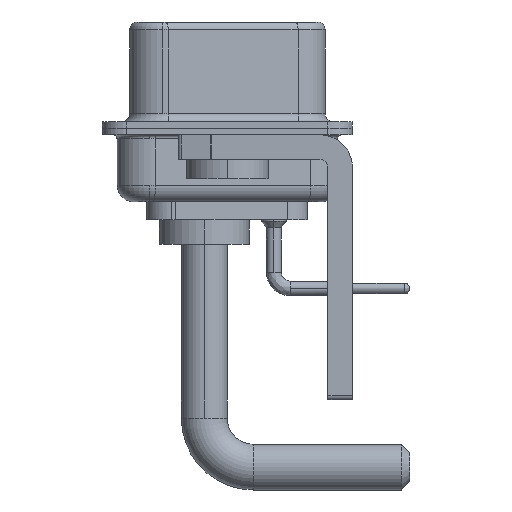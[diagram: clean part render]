
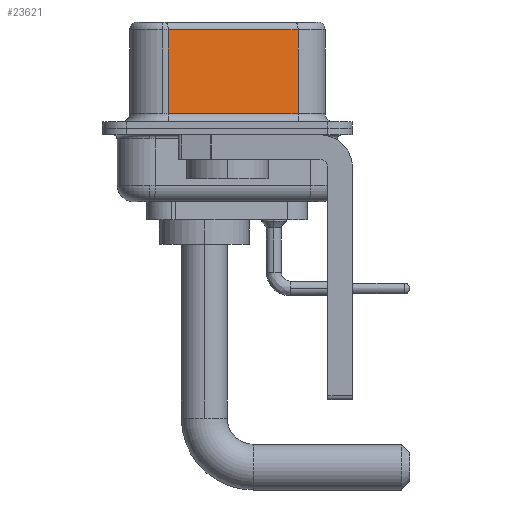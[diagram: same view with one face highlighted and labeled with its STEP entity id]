
A CAD part, left-side view. The second image highlights one B-rep face of the part: STEP entity #23621.
In plain terms, the highlighted planar face has unit normal (-0.985, -0.174, 0).
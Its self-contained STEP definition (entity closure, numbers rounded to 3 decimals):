
#509 = EDGE_CURVE ( 'NONE', #24397, #3879, #18357, .T. ) ;
#616 = CARTESIAN_POINT ( 'NONE',  ( 5.132, -4.322, 6.52 ) ) ;
#2607 = LINE ( 'NONE', #21674, #2951 ) ;
#2951 = VECTOR ( 'NONE', #10233, 1000. ) ;
#3073 = EDGE_CURVE ( 'NONE', #24397, #13013, #17763, .T. ) ;
#3879 = VERTEX_POINT ( 'NONE', #23460 ) ;
#5129 = DIRECTION ( 'NONE',  ( -0.174, 0.985, 0. ) ) ;
#5248 = CARTESIAN_POINT ( 'NONE',  ( 5.132, -4.322, 6.02 ) ) ;
#5534 = DIRECTION ( 'NONE',  ( 0., 0., -1. ) ) ;
#6666 = VECTOR ( 'NONE', #5129, 1000. ) ;
#7644 = CARTESIAN_POINT ( 'NONE',  ( 3.73, 3.628, 6.52 ) ) ;
#7901 = VECTOR ( 'NONE', #5534, 1000. ) ;
#8157 = ORIENTED_EDGE ( 'NONE', *, *, #509, .T. ) ;
#8603 = CARTESIAN_POINT ( 'NONE',  ( 5.132, -4.322, 0.9 ) ) ;
#8663 = VECTOR ( 'NONE', #21940, 1000. ) ;
#8993 = CARTESIAN_POINT ( 'NONE',  ( 5.132, -4.322, 6.02 ) ) ;
#9545 = CARTESIAN_POINT ( 'NONE',  ( 5.132, -4.322, 6.52 ) ) ;
#10233 = DIRECTION ( 'NONE',  ( 0.174, -0.985, 0. ) ) ;
#11800 = DIRECTION ( 'NONE',  ( -0.174, 0.985, 0. ) ) ;
#13013 = VERTEX_POINT ( 'NONE', #8603 ) ;
#13228 = VERTEX_POINT ( 'NONE', #14570 ) ;
#14570 = CARTESIAN_POINT ( 'NONE',  ( 3.73, 3.628, 0.9 ) ) ;
#15172 = PLANE ( 'NONE',  #15456 ) ;
#15456 = AXIS2_PLACEMENT_3D ( 'NONE', #9545, #19810, #11800 ) ;
#17763 = LINE ( 'NONE', #616, #8663 ) ;
#18357 = LINE ( 'NONE', #5248, #6666 ) ;
#18931 = FACE_OUTER_BOUND ( 'NONE', #23311, .T. ) ;
#19079 = EDGE_CURVE ( 'NONE', #13228, #13013, #2607, .T. ) ;
#19740 = ORIENTED_EDGE ( 'NONE', *, *, #3073, .F. ) ;
#19810 = DIRECTION ( 'NONE',  ( 0.985, 0.174, 0. ) ) ;
#20903 = ORIENTED_EDGE ( 'NONE', *, *, #19079, .T. ) ;
#20919 = ORIENTED_EDGE ( 'NONE', *, *, #24064, .T. ) ;
#21674 = CARTESIAN_POINT ( 'NONE',  ( 5.132, -4.322, 0.9 ) ) ;
#21940 = DIRECTION ( 'NONE',  ( 0., 0., -1. ) ) ;
#22718 = LINE ( 'NONE', #7644, #7901 ) ;
#23311 = EDGE_LOOP ( 'NONE', ( #19740, #8157, #20919, #20903 ) ) ;
#23460 = CARTESIAN_POINT ( 'NONE',  ( 3.73, 3.628, 6.02 ) ) ;
#23621 = ADVANCED_FACE ( 'NONE', ( #18931 ), #15172, .F. ) ;
#24064 = EDGE_CURVE ( 'NONE', #3879, #13228, #22718, .T. ) ;
#24397 = VERTEX_POINT ( 'NONE', #8993 ) ;
